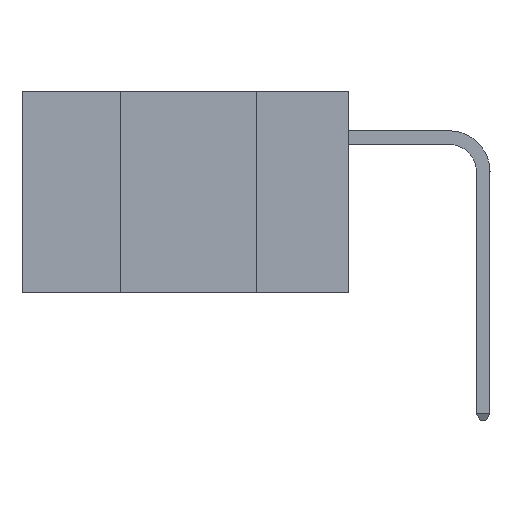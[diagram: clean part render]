
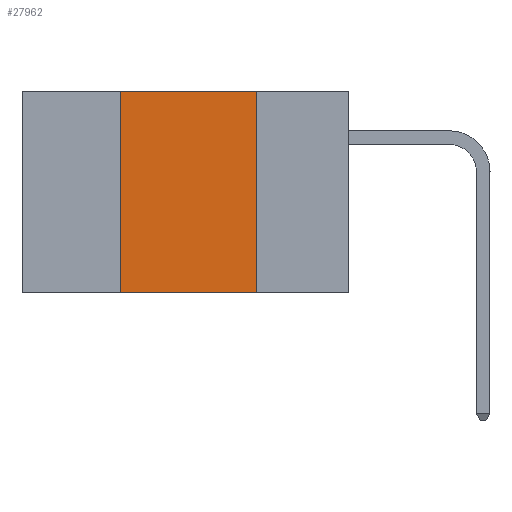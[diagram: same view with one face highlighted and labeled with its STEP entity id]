
A CAD part, left-side view. The second image highlights one B-rep face of the part: STEP entity #27962.
In plain terms, the highlighted planar face has unit normal (-1, 0, 0).
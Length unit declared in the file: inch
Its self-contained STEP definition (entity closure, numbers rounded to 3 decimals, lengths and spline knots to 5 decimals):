
#1399 = VERTEX_POINT ( 'NONE', #13099 ) ;
#2016 = EDGE_CURVE ( 'NONE', #10668, #1399, #3691, .T. ) ;
#3691 = LINE ( 'NONE', #24569, #33261 ) ;
#4160 = VECTOR ( 'NONE', #29708, 39.37008 ) ;
#5751 = ORIENTED_EDGE ( 'NONE', *, *, #29804, .F. ) ;
#6084 = EDGE_CURVE ( 'NONE', #1399, #11762, #26955, .T. ) ;
#8046 = CARTESIAN_POINT ( 'NONE',  ( 0., 0.17, -0.37 ) ) ;
#10668 = VERTEX_POINT ( 'NONE', #36875 ) ;
#11403 = EDGE_LOOP ( 'NONE', ( #23789, #17125, #5751, #22387 ) ) ;
#11762 = VERTEX_POINT ( 'NONE', #8046 ) ;
#13099 = CARTESIAN_POINT ( 'NONE',  ( 0., 0.17, 0. ) ) ;
#17125 = ORIENTED_EDGE ( 'NONE', *, *, #2016, .F. ) ;
#18582 = DIRECTION ( 'NONE',  ( 0., 0., -1. ) ) ;
#18901 = DIRECTION ( 'NONE',  ( 0., 0., -1. ) ) ;
#22387 = ORIENTED_EDGE ( 'NONE', *, *, #27924, .T. ) ;
#22657 = VECTOR ( 'NONE', #32667, 39.37008 ) ;
#23534 = LINE ( 'NONE', #27127, #22657 ) ;
#23789 = ORIENTED_EDGE ( 'NONE', *, *, #6084, .F. ) ;
#24569 = CARTESIAN_POINT ( 'NONE',  ( 0., 0.6, 0. ) ) ;
#24598 = CARTESIAN_POINT ( 'NONE',  ( 0., 0.17, 0. ) ) ;
#26060 = VECTOR ( 'NONE', #18901, 39.37008 ) ;
#26864 = CARTESIAN_POINT ( 'NONE',  ( 0., 0.6, -0.37 ) ) ;
#26955 = LINE ( 'NONE', #24598, #26060 ) ;
#27088 = LINE ( 'NONE', #26864, #4160 ) ;
#27127 = CARTESIAN_POINT ( 'NONE',  ( 0., 0.42, 0. ) ) ;
#27924 = EDGE_CURVE ( 'NONE', #36527, #11762, #27088, .T. ) ;
#27962 = ADVANCED_FACE ( 'NONE', ( #32816 ), #32659, .F. ) ;
#29708 = DIRECTION ( 'NONE',  ( 0., -1., 0. ) ) ;
#29804 = EDGE_CURVE ( 'NONE', #36527, #10668, #23534, .T. ) ;
#29833 = CARTESIAN_POINT ( 'NONE',  ( 0., 0.6, 0. ) ) ;
#30235 = DIRECTION ( 'NONE',  ( 0., -1., 0. ) ) ;
#32237 = CARTESIAN_POINT ( 'NONE',  ( 0., 0.42, -0.37 ) ) ;
#32659 = PLANE ( 'NONE',  #35752 ) ;
#32667 = DIRECTION ( 'NONE',  ( 0., 0., 1. ) ) ;
#32816 = FACE_OUTER_BOUND ( 'NONE', #11403, .T. ) ;
#33261 = VECTOR ( 'NONE', #30235, 39.37008 ) ;
#35522 = DIRECTION ( 'NONE',  ( 1., 0., 0. ) ) ;
#35752 = AXIS2_PLACEMENT_3D ( 'NONE', #29833, #35522, #18582 ) ;
#36527 = VERTEX_POINT ( 'NONE', #32237 ) ;
#36875 = CARTESIAN_POINT ( 'NONE',  ( 0., 0.42, 0. ) ) ;
